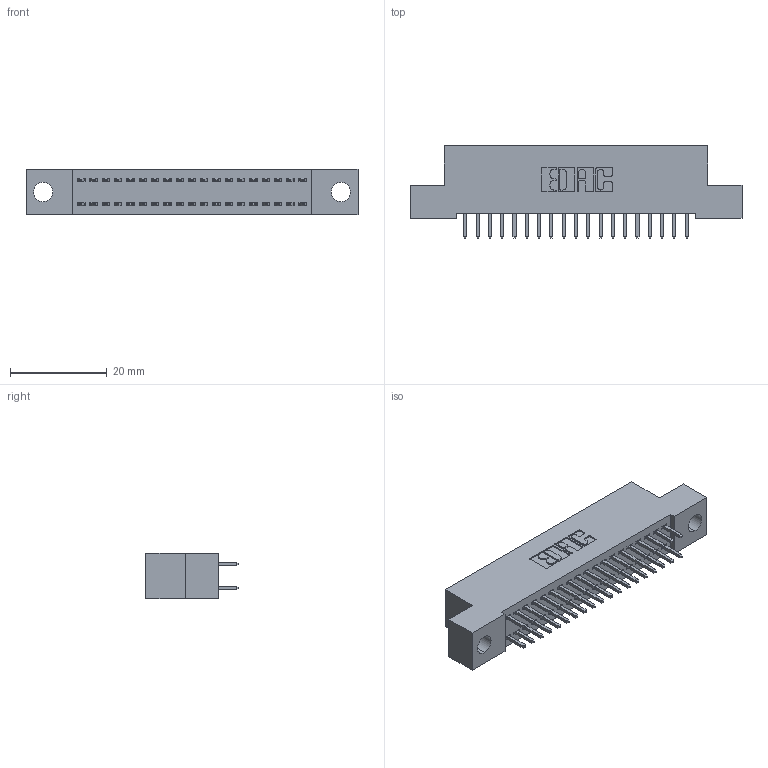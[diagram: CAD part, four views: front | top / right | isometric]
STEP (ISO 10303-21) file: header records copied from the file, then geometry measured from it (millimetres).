
FILE_DESCRIPTION (( 'STEP AP203' ), '1' );
FILE_NAME ('342-038-521-204.STEP', '2018-08-11T21:55:00', ( '' ), ( '' ), 'SwSTEP 2.0', 'SolidWorks 2016', '' );
FILE_SCHEMA (( 'CONFIG_CONTROL_DESIGN' ));
Length unit declared in the file: inch
Products named in the file (3): 342 Part_.156 TH; 345-292-001_345-293-121; 342-038-521-204
Assembly tree (39 placements, depth 2):
  342-038-521-204
    342 Part_.156 TH
    345-292-001_345-293-121  x38
Bounding box: 68.58 x 19.06 x 9.4 mm (x, y, z)
Volume: 5950.5 mm3; surface area: 8838.4 mm2
Topology: 39 solids, 39 shells, 2086 faces, 6189 edges, 4074 vertices
Faces by surface type: plane 1434, cylinder 652
Entity records: 15087 total; most frequent: CARTESIAN_POINT 2526, ORIENTED_EDGE 2462, DIRECTION 2199, EDGE_CURVE 1231, VECTOR 1103, LINE 1103, VERTEX_POINT 818, AXIS2_PLACEMENT_3D 548
